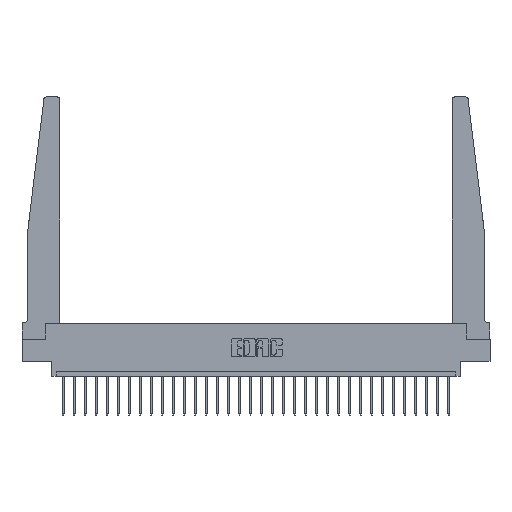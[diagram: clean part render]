
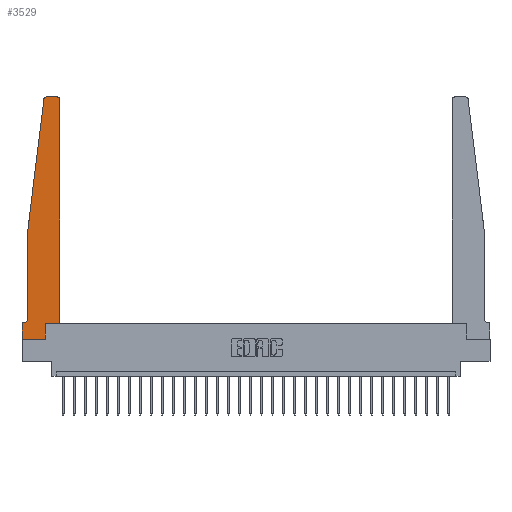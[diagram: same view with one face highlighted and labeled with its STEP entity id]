
A CAD part, top view. The second image highlights one B-rep face of the part: STEP entity #3529.
In plain terms, the highlighted planar face has unit normal (0, 0, 1).
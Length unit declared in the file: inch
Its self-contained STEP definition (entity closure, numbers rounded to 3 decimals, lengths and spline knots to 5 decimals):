
#563 = EDGE_CURVE ( 'NONE', #27530, #27613, #4637, .T. ) ;
#672 = VECTOR ( 'NONE', #26801, 39.37008 ) ;
#756 = EDGE_CURVE ( 'NONE', #22732, #5470, #20759, .T. ) ;
#1061 = VERTEX_POINT ( 'NONE', #25240 ) ;
#1135 = EDGE_CURVE ( 'NONE', #6835, #19461, #3562, .T. ) ;
#1159 = PLANE ( 'NONE',  #24070 ) ;
#1168 = ORIENTED_EDGE ( 'NONE', *, *, #6009, .T. ) ;
#1547 = CARTESIAN_POINT ( 'NONE',  ( 0.2605, 0., 0.37 ) ) ;
#1575 = CIRCLE ( 'NONE', #11657, 0.03 ) ;
#1629 = EDGE_CURVE ( 'NONE', #21183, #27530, #20348, .T. ) ;
#1654 = VECTOR ( 'NONE', #8327, 39.37008 ) ;
#1734 = CIRCLE ( 'NONE', #5410, 0.05 ) ;
#2594 = VERTEX_POINT ( 'NONE', #3540 ) ;
#3042 = DIRECTION ( 'NONE',  ( 0., 1., 0. ) ) ;
#3088 = LINE ( 'NONE', #11829, #24158 ) ;
#3111 = ORIENTED_EDGE ( 'NONE', *, *, #27475, .T. ) ;
#3529 = ADVANCED_FACE ( 'NONE', ( #5359 ), #1159, .T. ) ;
#3540 = CARTESIAN_POINT ( 'NONE',  ( 0.2605, 0.18, 0.37 ) ) ;
#3562 = LINE ( 'NONE', #23649, #1654 ) ;
#3886 = CARTESIAN_POINT ( 'NONE',  ( 0.395, 2.72, 0.37 ) ) ;
#4201 = EDGE_CURVE ( 'NONE', #5470, #1061, #21196, .T. ) ;
#4469 = VERTEX_POINT ( 'NONE', #25527 ) ;
#4637 = LINE ( 'NONE', #10933, #19139 ) ;
#4727 = CARTESIAN_POINT ( 'NONE',  ( 0., 0., 0.37 ) ) ;
#4844 = ORIENTED_EDGE ( 'NONE', *, *, #23285, .T. ) ;
#4900 = ORIENTED_EDGE ( 'NONE', *, *, #756, .T. ) ;
#4956 = EDGE_CURVE ( 'NONE', #23360, #2594, #25282, .T. ) ;
#5006 = VECTOR ( 'NONE', #7088, 39.37008 ) ;
#5059 = DIRECTION ( 'NONE',  ( 0., -1., 0. ) ) ;
#5322 = DIRECTION ( 'NONE',  ( -0.122, -0.992, 0. ) ) ;
#5359 = FACE_OUTER_BOUND ( 'NONE', #22722, .T. ) ;
#5410 = AXIS2_PLACEMENT_3D ( 'NONE', #25350, #5538, #12126 ) ;
#5413 = EDGE_CURVE ( 'NONE', #1061, #21183, #1734, .T. ) ;
#5470 = VERTEX_POINT ( 'NONE', #21121 ) ;
#5538 = DIRECTION ( 'NONE',  ( 0., 0., -1. ) ) ;
#5815 = ORIENTED_EDGE ( 'NONE', *, *, #4956, .T. ) ;
#5916 = CARTESIAN_POINT ( 'NONE',  ( 0.015, 0.1875, 0.37 ) ) ;
#6009 = EDGE_CURVE ( 'NONE', #27613, #23360, #11479, .T. ) ;
#6104 = CARTESIAN_POINT ( 'NONE',  ( 0.24675, 2.72367, 0.37 ) ) ;
#6653 = DIRECTION ( 'NONE',  ( 0., 0., 1. ) ) ;
#6835 = VERTEX_POINT ( 'NONE', #11735 ) ;
#7088 = DIRECTION ( 'NONE',  ( -1., 0., 0. ) ) ;
#8327 = DIRECTION ( 'NONE',  ( 0., 1., 0. ) ) ;
#9887 = CIRCLE ( 'NONE', #13577, 0.03 ) ;
#9888 = DIRECTION ( 'NONE',  ( 1., 0., 0. ) ) ;
#10050 = CARTESIAN_POINT ( 'NONE',  ( 0.065, 1.25, 0.37 ) ) ;
#10187 = ORIENTED_EDGE ( 'NONE', *, *, #23714, .T. ) ;
#10933 = CARTESIAN_POINT ( 'NONE',  ( 0., 0., 0.37 ) ) ;
#11479 = LINE ( 'NONE', #26045, #22520 ) ;
#11555 = LINE ( 'NONE', #15798, #672 ) ;
#11657 = AXIS2_PLACEMENT_3D ( 'NONE', #27282, #20745, #9888 ) ;
#11735 = CARTESIAN_POINT ( 'NONE',  ( 0.425, 0.18, 0.37 ) ) ;
#11829 = CARTESIAN_POINT ( 'NONE',  ( 0.425, 0.18, 0.37 ) ) ;
#12126 = DIRECTION ( 'NONE',  ( -1., 0., 0. ) ) ;
#12331 = ORIENTED_EDGE ( 'NONE', *, *, #1135, .T. ) ;
#12568 = ORIENTED_EDGE ( 'NONE', *, *, #563, .T. ) ;
#12853 = CARTESIAN_POINT ( 'NONE',  ( 0.395, 2.75, 0.37 ) ) ;
#13577 = AXIS2_PLACEMENT_3D ( 'NONE', #3886, #21452, #17106 ) ;
#14401 = VECTOR ( 'NONE', #3042, 39.37008 ) ;
#14696 = ORIENTED_EDGE ( 'NONE', *, *, #1629, .T. ) ;
#14717 = DIRECTION ( 'NONE',  ( 0., -1., 0. ) ) ;
#14787 = DIRECTION ( 'NONE',  ( 1., 0., 0. ) ) ;
#15255 = CARTESIAN_POINT ( 'NONE',  ( 0., 0.1875, 0.37 ) ) ;
#15798 = CARTESIAN_POINT ( 'NONE',  ( 0.25, 2.75, 0.37 ) ) ;
#16710 = CARTESIAN_POINT ( 'NONE',  ( 0.2605, 0.18, 0.37 ) ) ;
#17106 = DIRECTION ( 'NONE',  ( 1., 0., 0. ) ) ;
#18202 = CARTESIAN_POINT ( 'NONE',  ( 0.425, 2.72, 0.37 ) ) ;
#18403 = VERTEX_POINT ( 'NONE', #12853 ) ;
#19139 = VECTOR ( 'NONE', #5059, 39.37008 ) ;
#19461 = VERTEX_POINT ( 'NONE', #18202 ) ;
#20321 = DIRECTION ( 'NONE',  ( 1., 0., 0. ) ) ;
#20348 = LINE ( 'NONE', #20485, #5006 ) ;
#20485 = CARTESIAN_POINT ( 'NONE',  ( 0.065, 0.1875, 0.37 ) ) ;
#20731 = ORIENTED_EDGE ( 'NONE', *, *, #4201, .T. ) ;
#20745 = DIRECTION ( 'NONE',  ( 0., 0., 1. ) ) ;
#20759 = LINE ( 'NONE', #10050, #24262 ) ;
#21121 = CARTESIAN_POINT ( 'NONE',  ( 0.065, 1.25, 0.37 ) ) ;
#21183 = VERTEX_POINT ( 'NONE', #5916 ) ;
#21196 = LINE ( 'NONE', #27827, #24538 ) ;
#21452 = DIRECTION ( 'NONE',  ( 0., 0., 1. ) ) ;
#21529 = DIRECTION ( 'NONE',  ( 1., 0., 0. ) ) ;
#22520 = VECTOR ( 'NONE', #20321, 39.37008 ) ;
#22722 = EDGE_LOOP ( 'NONE', ( #10187, #4844, #4900, #20731, #26188, #14696, #12568, #1168, #5815, #24819, #12331, #3111 ) ) ;
#22732 = VERTEX_POINT ( 'NONE', #6104 ) ;
#23285 = EDGE_CURVE ( 'NONE', #4469, #22732, #1575, .T. ) ;
#23360 = VERTEX_POINT ( 'NONE', #1547 ) ;
#23426 = CARTESIAN_POINT ( 'NONE',  ( 0., 0.1875, 0.37 ) ) ;
#23649 = CARTESIAN_POINT ( 'NONE',  ( 0.425, 0.18, 0.37 ) ) ;
#23714 = EDGE_CURVE ( 'NONE', #18403, #4469, #11555, .T. ) ;
#23854 = EDGE_CURVE ( 'NONE', #2594, #6835, #3088, .T. ) ;
#24070 = AXIS2_PLACEMENT_3D ( 'NONE', #23426, #6653, #21529 ) ;
#24158 = VECTOR ( 'NONE', #14787, 39.37008 ) ;
#24262 = VECTOR ( 'NONE', #5322, 39.37008 ) ;
#24538 = VECTOR ( 'NONE', #14717, 39.37008 ) ;
#24819 = ORIENTED_EDGE ( 'NONE', *, *, #23854, .T. ) ;
#25240 = CARTESIAN_POINT ( 'NONE',  ( 0.065, 0.2375, 0.37 ) ) ;
#25282 = LINE ( 'NONE', #16710, #14401 ) ;
#25350 = CARTESIAN_POINT ( 'NONE',  ( 0.015, 0.2375, 0.37 ) ) ;
#25527 = CARTESIAN_POINT ( 'NONE',  ( 0.27653, 2.75, 0.37 ) ) ;
#26045 = CARTESIAN_POINT ( 'NONE',  ( 0., 0., 0.37 ) ) ;
#26188 = ORIENTED_EDGE ( 'NONE', *, *, #5413, .T. ) ;
#26801 = DIRECTION ( 'NONE',  ( -1., 0., 0. ) ) ;
#27282 = CARTESIAN_POINT ( 'NONE',  ( 0.27653, 2.72, 0.37 ) ) ;
#27475 = EDGE_CURVE ( 'NONE', #19461, #18403, #9887, .T. ) ;
#27530 = VERTEX_POINT ( 'NONE', #15255 ) ;
#27613 = VERTEX_POINT ( 'NONE', #4727 ) ;
#27827 = CARTESIAN_POINT ( 'NONE',  ( 0.065, 1.25, 0.37 ) ) ;
